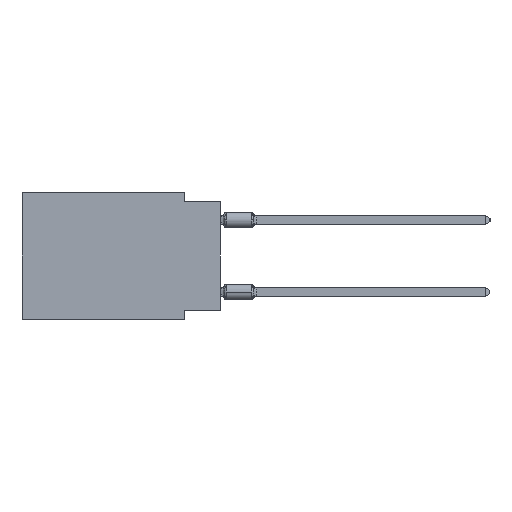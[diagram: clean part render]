
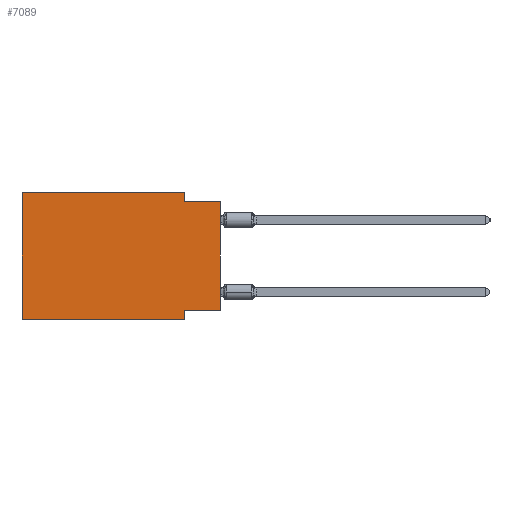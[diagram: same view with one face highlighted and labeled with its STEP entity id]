
A CAD part, left-side view. The second image highlights one B-rep face of the part: STEP entity #7089.
In plain terms, the highlighted planar face has unit normal (-1, 0, 0).
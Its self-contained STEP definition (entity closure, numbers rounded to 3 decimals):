
#104 = CARTESIAN_POINT ( 'NONE',  ( 0., 13.97, 0. ) ) ;
#1086 = VERTEX_POINT ( 'NONE', #39530 ) ;
#2416 = LINE ( 'NONE', #40831, #14732 ) ;
#2578 = EDGE_CURVE ( 'NONE', #11268, #12515, #24329, .T. ) ;
#2855 = DIRECTION ( 'NONE',  ( 0., 0., 1. ) ) ;
#3293 = VERTEX_POINT ( 'NONE', #4036 ) ;
#3785 = CARTESIAN_POINT ( 'NONE',  ( 0., 2.54, 0. ) ) ;
#4036 = CARTESIAN_POINT ( 'NONE',  ( 0., 0., -8.255 ) ) ;
#4474 = CARTESIAN_POINT ( 'NONE',  ( 0., 0., -0.635 ) ) ;
#4926 = DIRECTION ( 'NONE',  ( 0., -1., 0. ) ) ;
#5625 = LINE ( 'NONE', #19557, #40734 ) ;
#6201 = EDGE_CURVE ( 'NONE', #17652, #11268, #33179, .T. ) ;
#6885 = EDGE_LOOP ( 'NONE', ( #42078, #16213, #35192, #36239, #39426, #32815, #9461, #21441 ) ) ;
#7089 = ADVANCED_FACE ( 'NONE', ( #36991 ), #19386, .F. ) ;
#7658 = AXIS2_PLACEMENT_3D ( 'NONE', #9323, #23263, #9539 ) ;
#9323 = CARTESIAN_POINT ( 'NONE',  ( 0., 13.97, 0. ) ) ;
#9461 = ORIENTED_EDGE ( 'NONE', *, *, #17235, .F. ) ;
#9539 = DIRECTION ( 'NONE',  ( 0., 0., -1. ) ) ;
#10415 = LINE ( 'NONE', #3785, #41520 ) ;
#11199 = CARTESIAN_POINT ( 'NONE',  ( 0., 0., -0.635 ) ) ;
#11268 = VERTEX_POINT ( 'NONE', #21877 ) ;
#12379 = CARTESIAN_POINT ( 'NONE',  ( 0., 13.97, -8.89 ) ) ;
#12515 = VERTEX_POINT ( 'NONE', #40384 ) ;
#13781 = EDGE_CURVE ( 'NONE', #17652, #1086, #5625, .T. ) ;
#14086 = DIRECTION ( 'NONE',  ( 0., 0., -1. ) ) ;
#14732 = VECTOR ( 'NONE', #2855, 1000. ) ;
#16213 = ORIENTED_EDGE ( 'NONE', *, *, #23746, .F. ) ;
#17235 = EDGE_CURVE ( 'NONE', #39288, #1086, #30028, .T. ) ;
#17652 = VERTEX_POINT ( 'NONE', #12379 ) ;
#18551 = VECTOR ( 'NONE', #40055, 1000. ) ;
#19358 = LINE ( 'NONE', #33072, #24877 ) ;
#19386 = PLANE ( 'NONE',  #7658 ) ;
#19557 = CARTESIAN_POINT ( 'NONE',  ( 0., 13.97, -8.89 ) ) ;
#20169 = CARTESIAN_POINT ( 'NONE',  ( 0., 2.54, -8.89 ) ) ;
#20532 = VECTOR ( 'NONE', #30458, 1000. ) ;
#21441 = ORIENTED_EDGE ( 'NONE', *, *, #32574, .F. ) ;
#21877 = CARTESIAN_POINT ( 'NONE',  ( 0., 13.97, 0. ) ) ;
#23263 = DIRECTION ( 'NONE',  ( 1., 0., 0. ) ) ;
#23746 = EDGE_CURVE ( 'NONE', #26130, #34531, #24438, .T. ) ;
#24329 = LINE ( 'NONE', #104, #24989 ) ;
#24438 = LINE ( 'NONE', #4474, #29752 ) ;
#24877 = VECTOR ( 'NONE', #33301, 1000. ) ;
#24989 = VECTOR ( 'NONE', #28209, 1000. ) ;
#25665 = EDGE_CURVE ( 'NONE', #12515, #26130, #10415, .T. ) ;
#26130 = VERTEX_POINT ( 'NONE', #29259 ) ;
#28209 = DIRECTION ( 'NONE',  ( 0., -1., 0. ) ) ;
#29259 = CARTESIAN_POINT ( 'NONE',  ( 0., 2.54, -0.635 ) ) ;
#29752 = VECTOR ( 'NONE', #4926, 1000. ) ;
#30028 = LINE ( 'NONE', #20169, #20532 ) ;
#30458 = DIRECTION ( 'NONE',  ( 0., 0., -1. ) ) ;
#32055 = CARTESIAN_POINT ( 'NONE',  ( 0., 2.54, -8.255 ) ) ;
#32574 = EDGE_CURVE ( 'NONE', #3293, #39288, #19358, .T. ) ;
#32815 = ORIENTED_EDGE ( 'NONE', *, *, #13781, .T. ) ;
#33072 = CARTESIAN_POINT ( 'NONE',  ( 0., 0., -8.255 ) ) ;
#33179 = LINE ( 'NONE', #36379, #18551 ) ;
#33301 = DIRECTION ( 'NONE',  ( 0., 1., 0. ) ) ;
#33506 = DIRECTION ( 'NONE',  ( 0., -1., 0. ) ) ;
#34531 = VERTEX_POINT ( 'NONE', #11199 ) ;
#35192 = ORIENTED_EDGE ( 'NONE', *, *, #25665, .F. ) ;
#36239 = ORIENTED_EDGE ( 'NONE', *, *, #2578, .F. ) ;
#36379 = CARTESIAN_POINT ( 'NONE',  ( 0., 13.97, 0. ) ) ;
#36991 = FACE_OUTER_BOUND ( 'NONE', #6885, .T. ) ;
#38694 = EDGE_CURVE ( 'NONE', #3293, #34531, #2416, .T. ) ;
#39288 = VERTEX_POINT ( 'NONE', #32055 ) ;
#39426 = ORIENTED_EDGE ( 'NONE', *, *, #6201, .F. ) ;
#39530 = CARTESIAN_POINT ( 'NONE',  ( 0., 2.54, -8.89 ) ) ;
#40055 = DIRECTION ( 'NONE',  ( 0., 0., 1. ) ) ;
#40384 = CARTESIAN_POINT ( 'NONE',  ( 0., 2.54, 0. ) ) ;
#40734 = VECTOR ( 'NONE', #33506, 1000. ) ;
#40831 = CARTESIAN_POINT ( 'NONE',  ( 0., 0., 0. ) ) ;
#41520 = VECTOR ( 'NONE', #14086, 1000. ) ;
#42078 = ORIENTED_EDGE ( 'NONE', *, *, #38694, .T. ) ;
